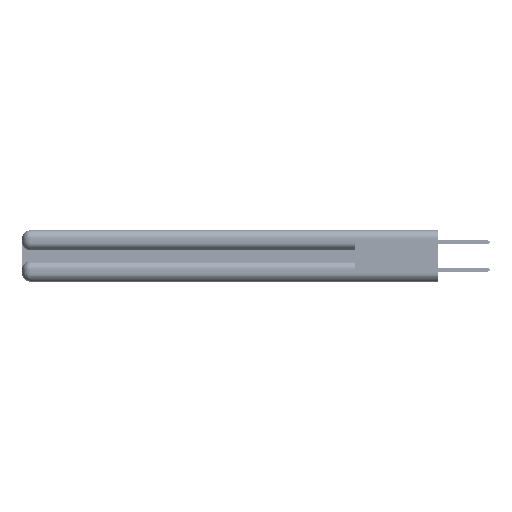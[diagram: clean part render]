
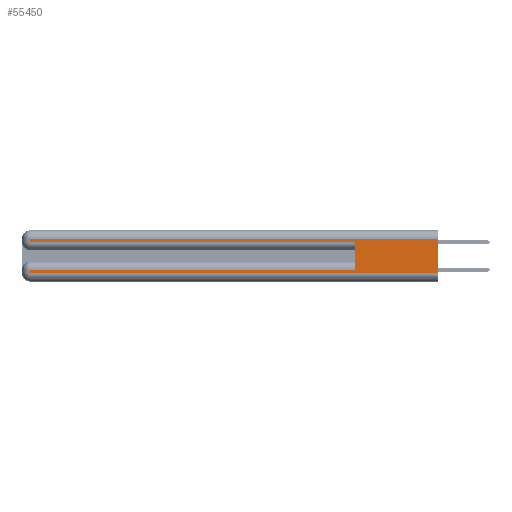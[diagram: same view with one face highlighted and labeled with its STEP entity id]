
A CAD part, left-side view. The second image highlights one B-rep face of the part: STEP entity #55450.
In plain terms, the highlighted planar face has unit normal (-1, 0, 0).
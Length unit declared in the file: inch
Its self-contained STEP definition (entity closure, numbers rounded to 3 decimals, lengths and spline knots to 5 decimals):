
#29 = VECTOR ( 'NONE', #51651, 39.37008 ) ;
#878 = CARTESIAN_POINT ( 'NONE',  ( 0., 0., 0.06 ) ) ;
#1842 = ORIENTED_EDGE ( 'NONE', *, *, #16050, .T. ) ;
#2718 = LINE ( 'NONE', #3917, #37870 ) ;
#3123 = EDGE_CURVE ( 'NONE', #37630, #53128, #28204, .T. ) ;
#3917 = CARTESIAN_POINT ( 'NONE',  ( 0., 0., 0.085 ) ) ;
#4296 = CARTESIAN_POINT ( 'NONE',  ( 0., 0., 0.31 ) ) ;
#4342 = LINE ( 'NONE', #32637, #13330 ) ;
#7312 = DIRECTION ( 'NONE',  ( 0., 1., 0. ) ) ;
#8167 = AXIS2_PLACEMENT_3D ( 'NONE', #21282, #52061, #25706 ) ;
#8561 = VECTOR ( 'NONE', #47593, 39.37008 ) ;
#12047 = EDGE_LOOP ( 'NONE', ( #21308, #13520, #31696, #12986, #33605, #1842, #19242, #55016 ) ) ;
#12197 = CARTESIAN_POINT ( 'NONE',  ( 0., 0., 0.37 ) ) ;
#12428 = DIRECTION ( 'NONE',  ( 0., 0., 1. ) ) ;
#12986 = ORIENTED_EDGE ( 'NONE', *, *, #26749, .T. ) ;
#13330 = VECTOR ( 'NONE', #41298, 39.37008 ) ;
#13520 = ORIENTED_EDGE ( 'NONE', *, *, #37467, .T. ) ;
#16050 = EDGE_CURVE ( 'NONE', #37630, #35935, #2718, .T. ) ;
#16490 = VECTOR ( 'NONE', #12428, 39.37008 ) ;
#16644 = CARTESIAN_POINT ( 'NONE',  ( 0., 0.6, 0.145 ) ) ;
#19180 = VECTOR ( 'NONE', #19844, 39.37008 ) ;
#19242 = ORIENTED_EDGE ( 'NONE', *, *, #49606, .T. ) ;
#19844 = DIRECTION ( 'NONE',  ( 0., -1., 0. ) ) ;
#20272 = LINE ( 'NONE', #12197, #8561 ) ;
#20605 = CARTESIAN_POINT ( 'NONE',  ( 0., 0., 0.31 ) ) ;
#20696 = LINE ( 'NONE', #20605, #42728 ) ;
#21186 = EDGE_CURVE ( 'NONE', #49153, #42636, #54308, .T. ) ;
#21282 = CARTESIAN_POINT ( 'NONE',  ( 0., 0., 0.37 ) ) ;
#21308 = ORIENTED_EDGE ( 'NONE', *, *, #24581, .F. ) ;
#21480 = CARTESIAN_POINT ( 'NONE',  ( 0., 2.94, 0.06 ) ) ;
#24581 = EDGE_CURVE ( 'NONE', #26154, #42636, #20272, .T. ) ;
#25706 = DIRECTION ( 'NONE',  ( 0., 0., -1. ) ) ;
#26154 = VERTEX_POINT ( 'NONE', #4296 ) ;
#26749 = EDGE_CURVE ( 'NONE', #26760, #53128, #47539, .T. ) ;
#26760 = VERTEX_POINT ( 'NONE', #52166 ) ;
#26777 = CARTESIAN_POINT ( 'NONE',  ( 0., 2.94, 0.31 ) ) ;
#28204 = LINE ( 'NONE', #16644, #16490 ) ;
#28705 = CARTESIAN_POINT ( 'NONE',  ( 0., 0., 0.06 ) ) ;
#28948 = CARTESIAN_POINT ( 'NONE',  ( 0., 0.6, 0.085 ) ) ;
#31696 = ORIENTED_EDGE ( 'NONE', *, *, #53308, .T. ) ;
#32637 = CARTESIAN_POINT ( 'NONE',  ( 0., 2.94, 0.37 ) ) ;
#33605 = ORIENTED_EDGE ( 'NONE', *, *, #3123, .F. ) ;
#34478 = DIRECTION ( 'NONE',  ( 0., -1., 0. ) ) ;
#35935 = VERTEX_POINT ( 'NONE', #36552 ) ;
#36552 = CARTESIAN_POINT ( 'NONE',  ( 0., 2.94, 0.085 ) ) ;
#36625 = LINE ( 'NONE', #42788, #29 ) ;
#37467 = EDGE_CURVE ( 'NONE', #26154, #52395, #20696, .T. ) ;
#37630 = VERTEX_POINT ( 'NONE', #28948 ) ;
#37870 = VECTOR ( 'NONE', #56643, 39.37008 ) ;
#38774 = PLANE ( 'NONE',  #8167 ) ;
#38883 = CARTESIAN_POINT ( 'NONE',  ( 0., 0., 0.285 ) ) ;
#41298 = DIRECTION ( 'NONE',  ( 0., 0., -1. ) ) ;
#42636 = VERTEX_POINT ( 'NONE', #878 ) ;
#42728 = VECTOR ( 'NONE', #7312, 39.37008 ) ;
#42788 = CARTESIAN_POINT ( 'NONE',  ( 0., 2.94, 0.37 ) ) ;
#44569 = CARTESIAN_POINT ( 'NONE',  ( 0., 0.6, 0.285 ) ) ;
#44719 = FACE_OUTER_BOUND ( 'NONE', #12047, .T. ) ;
#46156 = VECTOR ( 'NONE', #34478, 39.37008 ) ;
#47539 = LINE ( 'NONE', #38883, #46156 ) ;
#47593 = DIRECTION ( 'NONE',  ( 0., 0., -1. ) ) ;
#49153 = VERTEX_POINT ( 'NONE', #21480 ) ;
#49606 = EDGE_CURVE ( 'NONE', #35935, #49153, #36625, .T. ) ;
#51651 = DIRECTION ( 'NONE',  ( 0., 0., -1. ) ) ;
#52061 = DIRECTION ( 'NONE',  ( 1., 0., 0. ) ) ;
#52166 = CARTESIAN_POINT ( 'NONE',  ( 0., 2.94, 0.285 ) ) ;
#52395 = VERTEX_POINT ( 'NONE', #26777 ) ;
#53128 = VERTEX_POINT ( 'NONE', #44569 ) ;
#53308 = EDGE_CURVE ( 'NONE', #52395, #26760, #4342, .T. ) ;
#54308 = LINE ( 'NONE', #28705, #19180 ) ;
#55016 = ORIENTED_EDGE ( 'NONE', *, *, #21186, .T. ) ;
#55450 = ADVANCED_FACE ( 'NONE', ( #44719 ), #38774, .F. ) ;
#56643 = DIRECTION ( 'NONE',  ( 0., 1., 0. ) ) ;
